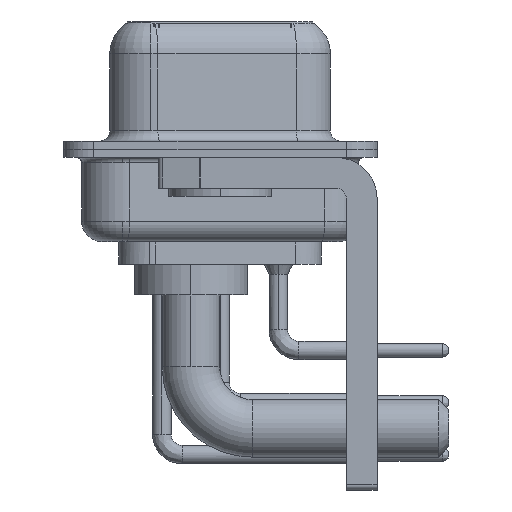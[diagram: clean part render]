
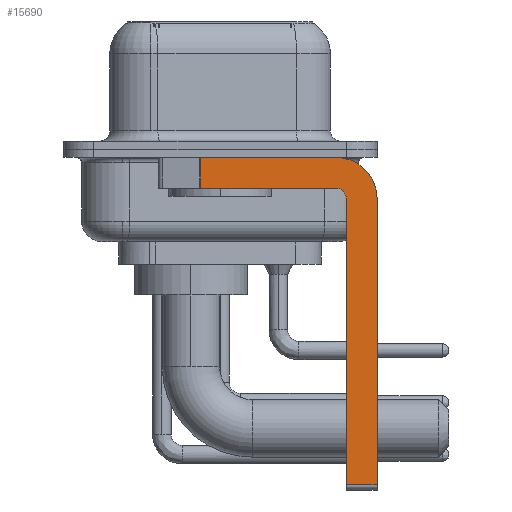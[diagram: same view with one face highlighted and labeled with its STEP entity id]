
A CAD part, left-side view. The second image highlights one B-rep face of the part: STEP entity #15690.
In plain terms, the highlighted planar face has unit normal (-1, 0, 0).
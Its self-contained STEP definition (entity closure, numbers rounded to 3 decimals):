
#562 = CARTESIAN_POINT ( 'NONE',  ( -2.9, -6.15, -16.35 ) ) ;
#1661 = CARTESIAN_POINT ( 'NONE',  ( -2.9, -5.65, -16.35 ) ) ;
#2389 = AXIS2_PLACEMENT_3D ( 'NONE', #31812, #26390, #13221 ) ;
#2493 = LINE ( 'NONE', #16340, #18485 ) ;
#2999 = CARTESIAN_POINT ( 'NONE',  ( -2.9, -5.65, -0.4 ) ) ;
#3128 = VERTEX_POINT ( 'NONE', #31476 ) ;
#3317 = EDGE_CURVE ( 'NONE', #12232, #3128, #21514, .T. ) ;
#3723 = EDGE_CURVE ( 'NONE', #19099, #12232, #26197, .T. ) ;
#4057 = VERTEX_POINT ( 'NONE', #30884 ) ;
#4156 = EDGE_CURVE ( 'NONE', #3128, #4057, #25802, .T. ) ;
#4212 = CARTESIAN_POINT ( 'NONE',  ( -2.9, 0.978, -1.9 ) ) ;
#4700 = AXIS2_PLACEMENT_3D ( 'NONE', #18850, #31648, #34290 ) ;
#5100 = CARTESIAN_POINT ( 'NONE',  ( -2.9, -6.15, -16.6 ) ) ;
#5817 = ORIENTED_EDGE ( 'NONE', *, *, #28059, .T. ) ;
#6404 = VECTOR ( 'NONE', #34182, 1000. ) ;
#6741 = LINE ( 'NONE', #1661, #33672 ) ;
#7331 = EDGE_CURVE ( 'NONE', #26120, #28573, #28577, .T. ) ;
#7418 = AXIS2_PLACEMENT_3D ( 'NONE', #10317, #26309, #15595 ) ;
#10317 = CARTESIAN_POINT ( 'NONE',  ( -2.9, -5.65, -2.4 ) ) ;
#10630 = ORIENTED_EDGE ( 'NONE', *, *, #21295, .T. ) ;
#11100 = VERTEX_POINT ( 'NONE', #12368 ) ;
#12232 = VERTEX_POINT ( 'NONE', #16464 ) ;
#12368 = CARTESIAN_POINT ( 'NONE',  ( -2.9, 0.978, -0.4 ) ) ;
#12456 = DIRECTION ( 'NONE',  ( 0., 1., 0. ) ) ;
#13075 = EDGE_CURVE ( 'NONE', #11100, #32999, #2493, .T. ) ;
#13221 = DIRECTION ( 'NONE',  ( 0., 0., -1. ) ) ;
#13296 = LINE ( 'NONE', #4212, #6404 ) ;
#13840 = ORIENTED_EDGE ( 'NONE', *, *, #4156, .F. ) ;
#14012 = ORIENTED_EDGE ( 'NONE', *, *, #3723, .F. ) ;
#14262 = VECTOR ( 'NONE', #12456, 1000. ) ;
#15595 = DIRECTION ( 'NONE',  ( 0., 0., -1. ) ) ;
#15690 = ADVANCED_FACE ( 'NONE', ( #23499 ), #25617, .F. ) ;
#15755 = DIRECTION ( 'NONE',  ( 0., 0., -1. ) ) ;
#16340 = CARTESIAN_POINT ( 'NONE',  ( -2.9, 3., -0.4 ) ) ;
#16464 = CARTESIAN_POINT ( 'NONE',  ( -2.9, -6.15, -2.4 ) ) ;
#16913 = EDGE_CURVE ( 'NONE', #32999, #26120, #18075, .T. ) ;
#18075 = CIRCLE ( 'NONE', #2389, 2. ) ;
#18106 = DIRECTION ( 'NONE',  ( 0., 0., 1. ) ) ;
#18485 = VECTOR ( 'NONE', #34614, 1000. ) ;
#18850 = CARTESIAN_POINT ( 'NONE',  ( -2.9, -5.65, -2.4 ) ) ;
#19099 = VERTEX_POINT ( 'NONE', #562 ) ;
#20567 = VECTOR ( 'NONE', #15755, 1000. ) ;
#21295 = EDGE_CURVE ( 'NONE', #11100, #4057, #13296, .T. ) ;
#21514 = CIRCLE ( 'NONE', #4700, 0.5 ) ;
#23021 = ORIENTED_EDGE ( 'NONE', *, *, #13075, .F. ) ;
#23120 = ORIENTED_EDGE ( 'NONE', *, *, #7331, .F. ) ;
#23499 = FACE_OUTER_BOUND ( 'NONE', #29642, .T. ) ;
#24560 = CARTESIAN_POINT ( 'NONE',  ( -2.9, -7.65, -2.4 ) ) ;
#25617 = PLANE ( 'NONE',  #7418 ) ;
#25802 = LINE ( 'NONE', #30522, #14262 ) ;
#26120 = VERTEX_POINT ( 'NONE', #24560 ) ;
#26197 = LINE ( 'NONE', #5100, #31062 ) ;
#26309 = DIRECTION ( 'NONE',  ( 1., 0., 0. ) ) ;
#26390 = DIRECTION ( 'NONE',  ( 1., 0., 0. ) ) ;
#28059 = EDGE_CURVE ( 'NONE', #19099, #28573, #6741, .T. ) ;
#28135 = CARTESIAN_POINT ( 'NONE',  ( -2.9, -7.65, -16.35 ) ) ;
#28573 = VERTEX_POINT ( 'NONE', #28135 ) ;
#28577 = LINE ( 'NONE', #34359, #20567 ) ;
#29642 = EDGE_LOOP ( 'NONE', ( #23021, #10630, #13840, #30918, #14012, #5817, #23120, #29661 ) ) ;
#29661 = ORIENTED_EDGE ( 'NONE', *, *, #16913, .F. ) ;
#30522 = CARTESIAN_POINT ( 'NONE',  ( -2.9, -5.65, -1.9 ) ) ;
#30884 = CARTESIAN_POINT ( 'NONE',  ( -2.9, 0.978, -1.9 ) ) ;
#30918 = ORIENTED_EDGE ( 'NONE', *, *, #3317, .F. ) ;
#30987 = DIRECTION ( 'NONE',  ( 0., -1., 0. ) ) ;
#31062 = VECTOR ( 'NONE', #18106, 1000. ) ;
#31476 = CARTESIAN_POINT ( 'NONE',  ( -2.9, -5.65, -1.9 ) ) ;
#31648 = DIRECTION ( 'NONE',  ( -1., 0., 0. ) ) ;
#31812 = CARTESIAN_POINT ( 'NONE',  ( -2.9, -5.65, -2.4 ) ) ;
#32999 = VERTEX_POINT ( 'NONE', #2999 ) ;
#33672 = VECTOR ( 'NONE', #30987, 1000. ) ;
#34182 = DIRECTION ( 'NONE',  ( 0., 0., -1. ) ) ;
#34290 = DIRECTION ( 'NONE',  ( 0., 0., 1. ) ) ;
#34359 = CARTESIAN_POINT ( 'NONE',  ( -2.9, -7.65, -2.4 ) ) ;
#34614 = DIRECTION ( 'NONE',  ( 0., -1., 0. ) ) ;
